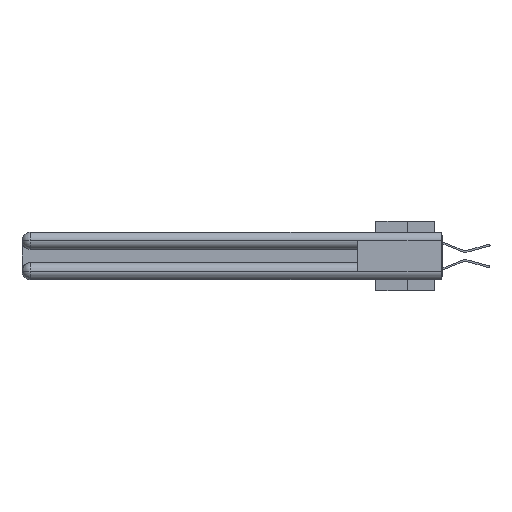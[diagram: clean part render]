
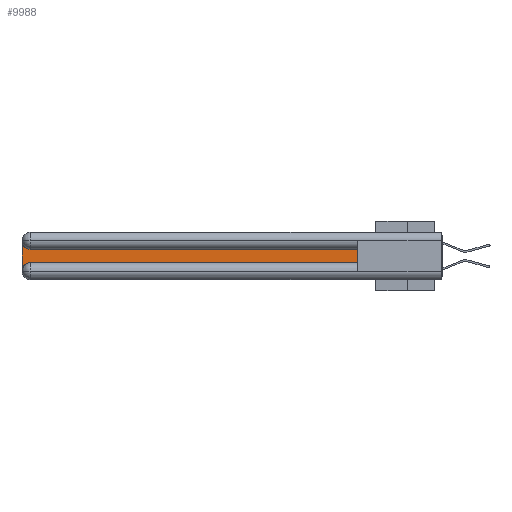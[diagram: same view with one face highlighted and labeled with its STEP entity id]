
A CAD part, left-side view. The second image highlights one B-rep face of the part: STEP entity #9988.
In plain terms, the highlighted planar face has unit normal (-1, 0, 0).
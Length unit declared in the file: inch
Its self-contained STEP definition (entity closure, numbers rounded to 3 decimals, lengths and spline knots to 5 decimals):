
#26 = VECTOR ( 'NONE', #23213, 39.37008 ) ;
#1117 = CARTESIAN_POINT ( 'NONE',  ( 0.075, 3., -0.0625 ) ) ;
#1140 = ORIENTED_EDGE ( 'NONE', *, *, #25882, .T. ) ;
#2276 = CARTESIAN_POINT ( 'NONE',  ( 0.075, 0.6, -0.2175 ) ) ;
#2429 = EDGE_CURVE ( 'NONE', #24432, #18782, #9067, .T. ) ;
#3045 = VECTOR ( 'NONE', #14003, 39.37008 ) ;
#3063 = EDGE_CURVE ( 'NONE', #11996, #32607, #10328, .T. ) ;
#5117 = ORIENTED_EDGE ( 'NONE', *, *, #2429, .T. ) ;
#5707 = EDGE_CURVE ( 'NONE', #30212, #24432, #33656, .T. ) ;
#6655 = AXIS2_PLACEMENT_3D ( 'NONE', #29941, #19819, #30465 ) ;
#6974 = EDGE_CURVE ( 'NONE', #32607, #30212, #13281, .T. ) ;
#7338 = AXIS2_PLACEMENT_3D ( 'NONE', #28969, #20761, #13336 ) ;
#8904 = VERTEX_POINT ( 'NONE', #2276 ) ;
#9067 = CIRCLE ( 'NONE', #11808, 0.06 ) ;
#9074 = ORIENTED_EDGE ( 'NONE', *, *, #5707, .T. ) ;
#9350 = ORIENTED_EDGE ( 'NONE', *, *, #6974, .T. ) ;
#9988 = ADVANCED_FACE ( 'NONE', ( #26230 ), #28457, .F. ) ;
#10105 = DIRECTION ( 'NONE',  ( 0., 0., -1. ) ) ;
#10328 = LINE ( 'NONE', #26134, #26 ) ;
#10427 = DIRECTION ( 'NONE',  ( 0., 0., 1. ) ) ;
#10460 = CARTESIAN_POINT ( 'NONE',  ( 0.075, 2.94, -0.2775 ) ) ;
#10607 = VECTOR ( 'NONE', #10427, 39.37008 ) ;
#11808 = AXIS2_PLACEMENT_3D ( 'NONE', #10460, #31109, #25926 ) ;
#11996 = VERTEX_POINT ( 'NONE', #19798 ) ;
#13281 = CIRCLE ( 'NONE', #6655, 0.06 ) ;
#13336 = DIRECTION ( 'NONE',  ( 0., 0., -1. ) ) ;
#14003 = DIRECTION ( 'NONE',  ( 0., -1., 0. ) ) ;
#16742 = EDGE_LOOP ( 'NONE', ( #29147, #9350, #9074, #5117, #24116, #1140 ) ) ;
#17344 = VECTOR ( 'NONE', #10105, 39.37008 ) ;
#18782 = VERTEX_POINT ( 'NONE', #20821 ) ;
#19263 = CARTESIAN_POINT ( 'NONE',  ( 0.075, 2.94, -0.1225 ) ) ;
#19798 = CARTESIAN_POINT ( 'NONE',  ( 0.075, 0.6, -0.1225 ) ) ;
#19819 = DIRECTION ( 'NONE',  ( 1., 0., 0. ) ) ;
#20761 = DIRECTION ( 'NONE',  ( 1., 0., 0. ) ) ;
#20774 = LINE ( 'NONE', #21275, #10607 ) ;
#20821 = CARTESIAN_POINT ( 'NONE',  ( 0.075, 2.94, -0.2175 ) ) ;
#21275 = CARTESIAN_POINT ( 'NONE',  ( 0.075, 0.6, -0.2175 ) ) ;
#22660 = EDGE_CURVE ( 'NONE', #18782, #8904, #32358, .T. ) ;
#22949 = CARTESIAN_POINT ( 'NONE',  ( 0.075, 3., -0.2775 ) ) ;
#23213 = DIRECTION ( 'NONE',  ( 0., 1., 0. ) ) ;
#24116 = ORIENTED_EDGE ( 'NONE', *, *, #22660, .T. ) ;
#24432 = VERTEX_POINT ( 'NONE', #22949 ) ;
#25569 = CARTESIAN_POINT ( 'NONE',  ( 0.075, 3., -0.2175 ) ) ;
#25882 = EDGE_CURVE ( 'NONE', #8904, #11996, #20774, .T. ) ;
#25926 = DIRECTION ( 'NONE',  ( 0., 0., -1. ) ) ;
#26134 = CARTESIAN_POINT ( 'NONE',  ( 0.075, 0.6, -0.1225 ) ) ;
#26230 = FACE_OUTER_BOUND ( 'NONE', #16742, .T. ) ;
#28457 = PLANE ( 'NONE',  #7338 ) ;
#28969 = CARTESIAN_POINT ( 'NONE',  ( 0.075, 3., -0.1225 ) ) ;
#29147 = ORIENTED_EDGE ( 'NONE', *, *, #3063, .T. ) ;
#29941 = CARTESIAN_POINT ( 'NONE',  ( 0.075, 2.94, -0.0625 ) ) ;
#29957 = CARTESIAN_POINT ( 'NONE',  ( 0.075, 0.6, -0.2175 ) ) ;
#30212 = VERTEX_POINT ( 'NONE', #1117 ) ;
#30465 = DIRECTION ( 'NONE',  ( 0., 0., -1. ) ) ;
#31109 = DIRECTION ( 'NONE',  ( 1., 0., 0. ) ) ;
#32358 = LINE ( 'NONE', #29957, #3045 ) ;
#32607 = VERTEX_POINT ( 'NONE', #19263 ) ;
#33656 = LINE ( 'NONE', #25569, #17344 ) ;
